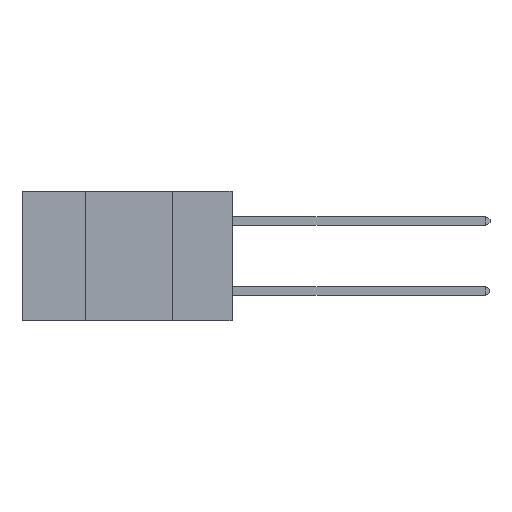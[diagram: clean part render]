
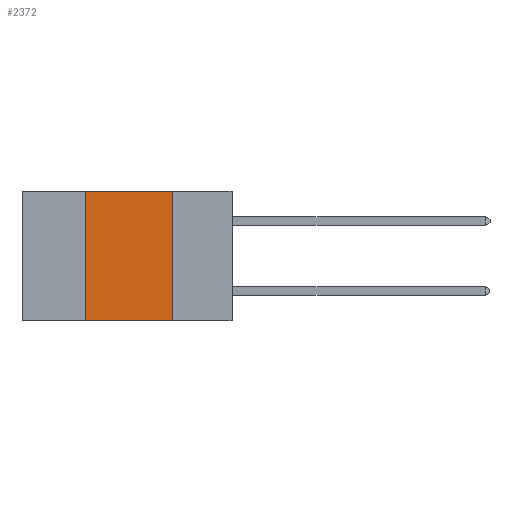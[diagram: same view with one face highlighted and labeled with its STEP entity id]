
A CAD part, left-side view. The second image highlights one B-rep face of the part: STEP entity #2372.
In plain terms, the highlighted planar face has unit normal (-1, 0, 0).
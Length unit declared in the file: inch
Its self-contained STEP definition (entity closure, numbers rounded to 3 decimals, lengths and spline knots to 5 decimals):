
#1065 = DIRECTION ( 'NONE',  ( 0., 0., -1. ) ) ;
#1470 = CARTESIAN_POINT ( 'NONE',  ( 0., 0.42, -0.37 ) ) ;
#1479 = VECTOR ( 'NONE', #6422, 39.37008 ) ;
#1636 = CARTESIAN_POINT ( 'NONE',  ( 0., 0.6, 0. ) ) ;
#2092 = CARTESIAN_POINT ( 'NONE',  ( 0., 0.42, 0. ) ) ;
#2283 = ORIENTED_EDGE ( 'NONE', *, *, #4484, .F. ) ;
#2372 = ADVANCED_FACE ( 'NONE', ( #7007 ), #8575, .F. ) ;
#2418 = EDGE_LOOP ( 'NONE', ( #2283, #13464, #7607, #3980 ) ) ;
#2676 = DIRECTION ( 'NONE',  ( 0., -1., 0. ) ) ;
#2919 = CARTESIAN_POINT ( 'NONE',  ( 0., 0.42, 0. ) ) ;
#3332 = AXIS2_PLACEMENT_3D ( 'NONE', #6912, #7980, #7345 ) ;
#3877 = LINE ( 'NONE', #1636, #6520 ) ;
#3980 = ORIENTED_EDGE ( 'NONE', *, *, #5953, .T. ) ;
#4364 = CARTESIAN_POINT ( 'NONE',  ( 0., 0.17, 0. ) ) ;
#4484 = EDGE_CURVE ( 'NONE', #6224, #5015, #5920, .T. ) ;
#5015 = VERTEX_POINT ( 'NONE', #11868 ) ;
#5156 = VECTOR ( 'NONE', #2676, 39.37008 ) ;
#5920 = LINE ( 'NONE', #9381, #13889 ) ;
#5953 = EDGE_CURVE ( 'NONE', #7228, #5015, #12883, .T. ) ;
#6224 = VERTEX_POINT ( 'NONE', #4364 ) ;
#6422 = DIRECTION ( 'NONE',  ( 0., 0., 1. ) ) ;
#6520 = VECTOR ( 'NONE', #8442, 39.37008 ) ;
#6717 = EDGE_CURVE ( 'NONE', #13877, #6224, #3877, .T. ) ;
#6912 = CARTESIAN_POINT ( 'NONE',  ( 0., 0.6, 0. ) ) ;
#7007 = FACE_OUTER_BOUND ( 'NONE', #2418, .T. ) ;
#7228 = VERTEX_POINT ( 'NONE', #1470 ) ;
#7345 = DIRECTION ( 'NONE',  ( 0., 0., -1. ) ) ;
#7607 = ORIENTED_EDGE ( 'NONE', *, *, #10618, .F. ) ;
#7980 = DIRECTION ( 'NONE',  ( 1., 0., 0. ) ) ;
#8258 = LINE ( 'NONE', #2919, #1479 ) ;
#8442 = DIRECTION ( 'NONE',  ( 0., -1., 0. ) ) ;
#8575 = PLANE ( 'NONE',  #3332 ) ;
#9302 = CARTESIAN_POINT ( 'NONE',  ( 0., 0.6, -0.37 ) ) ;
#9381 = CARTESIAN_POINT ( 'NONE',  ( 0., 0.17, 0. ) ) ;
#10618 = EDGE_CURVE ( 'NONE', #7228, #13877, #8258, .T. ) ;
#11868 = CARTESIAN_POINT ( 'NONE',  ( 0., 0.17, -0.37 ) ) ;
#12883 = LINE ( 'NONE', #9302, #5156 ) ;
#13464 = ORIENTED_EDGE ( 'NONE', *, *, #6717, .F. ) ;
#13877 = VERTEX_POINT ( 'NONE', #2092 ) ;
#13889 = VECTOR ( 'NONE', #1065, 39.37008 ) ;
